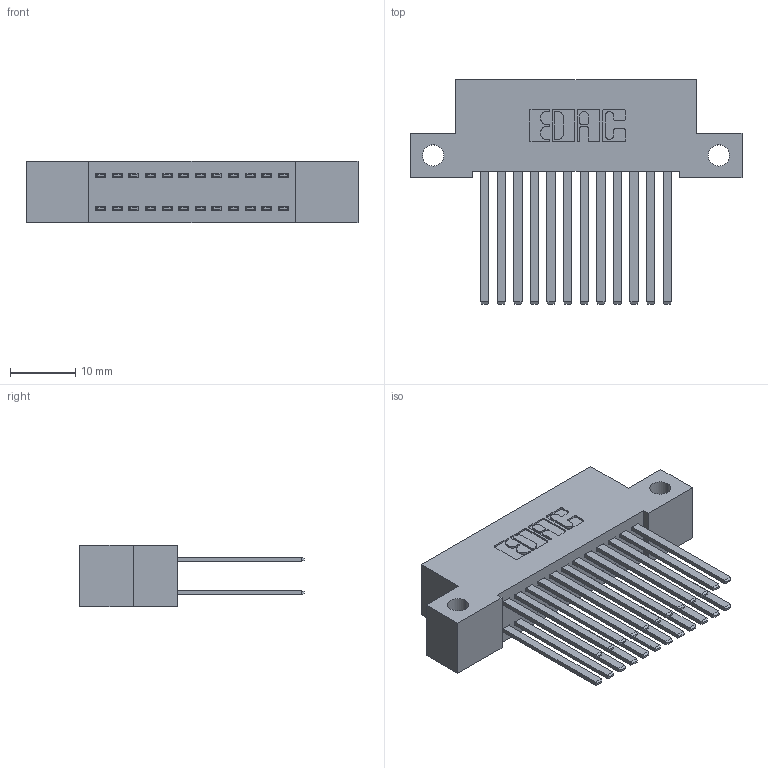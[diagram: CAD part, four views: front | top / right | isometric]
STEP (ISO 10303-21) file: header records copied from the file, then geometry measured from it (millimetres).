
FILE_DESCRIPTION (( 'STEP AP203' ), '1' );
FILE_NAME ('342-024-544-212.STEP', '2018-08-11T02:47:15', ( '' ), ( '' ), 'SwSTEP 2.0', 'SolidWorks 2016', '' );
FILE_SCHEMA (( 'CONFIG_CONTROL_DESIGN' ));
Length unit declared in the file: inch
Products named in the file (3): 342 Part_Side Mount; 345-292-001_345-293-144; 342-024-544-212
Assembly tree (25 placements, depth 2):
  342-024-544-212
    342 Part_Side Mount
    345-292-001_345-293-144  x24
Bounding box: 50.8 x 34.3 x 9.4 mm (x, y, z)
Volume: 4684.9 mm3; surface area: 7658.5 mm2
Topology: 25 solids, 25 shells, 1214 faces, 3587 edges, 2358 vertices
Faces by surface type: plane 834, cylinder 380
Entity records: 11287 total; most frequent: CARTESIAN_POINT 1902, ORIENTED_EDGE 1838, DIRECTION 1675, EDGE_CURVE 919, VECTOR 795, LINE 795, VERTEX_POINT 610, AXIS2_PLACEMENT_3D 440
